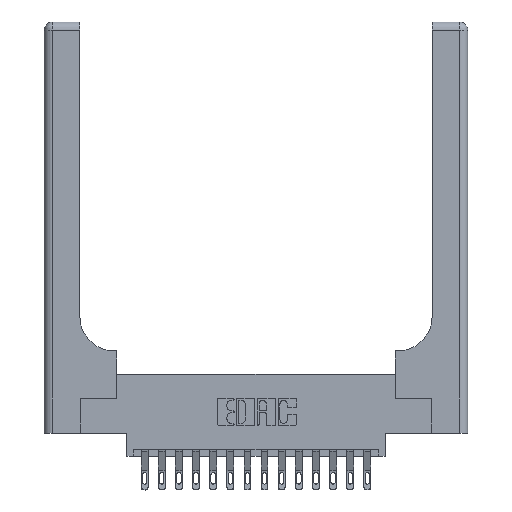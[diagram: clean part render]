
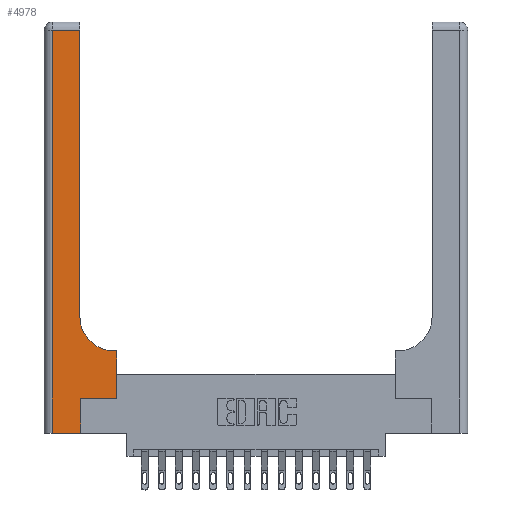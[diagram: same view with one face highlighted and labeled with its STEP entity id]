
A CAD part, top view. The second image highlights one B-rep face of the part: STEP entity #4978.
In plain terms, the highlighted planar face has unit normal (0, 0, 1).
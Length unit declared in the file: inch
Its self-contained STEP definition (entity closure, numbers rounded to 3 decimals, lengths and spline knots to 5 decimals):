
#12 = CARTESIAN_POINT ( 'NONE',  ( 0.26, 2.94, 0.37 ) ) ;
#31 = CARTESIAN_POINT ( 'NONE',  ( 0.26, 3., 0.37 ) ) ;
#469 = VERTEX_POINT ( 'NONE', #12 ) ;
#737 = ORIENTED_EDGE ( 'NONE', *, *, #15162, .T. ) ;
#1113 = VECTOR ( 'NONE', #2890, 39.37008 ) ;
#1508 = DIRECTION ( 'NONE',  ( 0., 1., 0. ) ) ;
#2030 = DIRECTION ( 'NONE',  ( -1., 0., 0. ) ) ;
#2580 = CARTESIAN_POINT ( 'NONE',  ( 0., 2.94, 0.37 ) ) ;
#2603 = VECTOR ( 'NONE', #15039, 39.37008 ) ;
#2890 = DIRECTION ( 'NONE',  ( 1., 0., 0. ) ) ;
#2992 = CARTESIAN_POINT ( 'NONE',  ( 0.528, 0.25, 0.37 ) ) ;
#3216 = VERTEX_POINT ( 'NONE', #11902 ) ;
#3473 = VERTEX_POINT ( 'NONE', #8165 ) ;
#3650 = EDGE_CURVE ( 'NONE', #15728, #469, #12330, .T. ) ;
#3864 = CARTESIAN_POINT ( 'NONE',  ( 0.26, 0.85, 0.37 ) ) ;
#4078 = VECTOR ( 'NONE', #12043, 39.37008 ) ;
#4079 = DIRECTION ( 'NONE',  ( -1., 0., 0. ) ) ;
#4214 = CARTESIAN_POINT ( 'NONE',  ( 0.528, 0.25, 0.37 ) ) ;
#4428 = VERTEX_POINT ( 'NONE', #9135 ) ;
#4525 = LINE ( 'NONE', #2580, #15442 ) ;
#4595 = AXIS2_PLACEMENT_3D ( 'NONE', #5331, #15278, #6759 ) ;
#4690 = PLANE ( 'NONE',  #7529 ) ;
#4805 = VECTOR ( 'NONE', #6976, 39.37008 ) ;
#4978 = ADVANCED_FACE ( 'NONE', ( #9402 ), #4690, .F. ) ;
#5121 = EDGE_CURVE ( 'NONE', #3216, #15539, #7165, .T. ) ;
#5331 = CARTESIAN_POINT ( 'NONE',  ( 0.51, 0.85, 0.37 ) ) ;
#5892 = EDGE_CURVE ( 'NONE', #11147, #3216, #17343, .T. ) ;
#5900 = ORIENTED_EDGE ( 'NONE', *, *, #14709, .T. ) ;
#6041 = VECTOR ( 'NONE', #11325, 39.37008 ) ;
#6281 = CARTESIAN_POINT ( 'NONE',  ( 0.51, 0.6, 0.37 ) ) ;
#6331 = CARTESIAN_POINT ( 'NONE',  ( 0.06, 3., 0.37 ) ) ;
#6537 = EDGE_CURVE ( 'NONE', #8228, #11248, #8812, .T. ) ;
#6759 = DIRECTION ( 'NONE',  ( 1., 0., 0. ) ) ;
#6817 = EDGE_CURVE ( 'NONE', #3473, #11147, #8582, .T. ) ;
#6976 = DIRECTION ( 'NONE',  ( 1., 0., 0. ) ) ;
#7165 = LINE ( 'NONE', #7799, #10519 ) ;
#7529 = AXIS2_PLACEMENT_3D ( 'NONE', #16071, #7547, #17464 ) ;
#7547 = DIRECTION ( 'NONE',  ( 0., 0., -1. ) ) ;
#7799 = CARTESIAN_POINT ( 'NONE',  ( 0.26, 0.6, 0.37 ) ) ;
#8065 = ORIENTED_EDGE ( 'NONE', *, *, #17404, .T. ) ;
#8165 = CARTESIAN_POINT ( 'NONE',  ( 0.265, 0.25, 0.37 ) ) ;
#8228 = VERTEX_POINT ( 'NONE', #14720 ) ;
#8582 = LINE ( 'NONE', #16906, #4805 ) ;
#8812 = LINE ( 'NONE', #15780, #1113 ) ;
#9135 = CARTESIAN_POINT ( 'NONE',  ( 0.06, 2.94, 0.37 ) ) ;
#9336 = CIRCLE ( 'NONE', #4595, 0.25 ) ;
#9402 = FACE_OUTER_BOUND ( 'NONE', #16044, .T. ) ;
#10519 = VECTOR ( 'NONE', #2030, 39.37008 ) ;
#11147 = VERTEX_POINT ( 'NONE', #2992 ) ;
#11229 = ORIENTED_EDGE ( 'NONE', *, *, #5892, .T. ) ;
#11248 = VERTEX_POINT ( 'NONE', #11810 ) ;
#11325 = DIRECTION ( 'NONE',  ( 0., 1., 0. ) ) ;
#11666 = LINE ( 'NONE', #6331, #4078 ) ;
#11810 = CARTESIAN_POINT ( 'NONE',  ( 0.265, 0., 0.37 ) ) ;
#11887 = VECTOR ( 'NONE', #1508, 39.37008 ) ;
#11902 = CARTESIAN_POINT ( 'NONE',  ( 0.528, 0.6, 0.37 ) ) ;
#11936 = EDGE_CURVE ( 'NONE', #15539, #15728, #9336, .T. ) ;
#12043 = DIRECTION ( 'NONE',  ( 0., -1., 0. ) ) ;
#12330 = LINE ( 'NONE', #31, #11887 ) ;
#13354 = ORIENTED_EDGE ( 'NONE', *, *, #11936, .T. ) ;
#13467 = ORIENTED_EDGE ( 'NONE', *, *, #5121, .T. ) ;
#14709 = EDGE_CURVE ( 'NONE', #4428, #8228, #11666, .T. ) ;
#14720 = CARTESIAN_POINT ( 'NONE',  ( 0.06, 0., 0.37 ) ) ;
#15039 = DIRECTION ( 'NONE',  ( 0., 1., 0. ) ) ;
#15162 = EDGE_CURVE ( 'NONE', #469, #4428, #4525, .T. ) ;
#15278 = DIRECTION ( 'NONE',  ( 0., 0., -1. ) ) ;
#15442 = VECTOR ( 'NONE', #4079, 39.37008 ) ;
#15539 = VERTEX_POINT ( 'NONE', #6281 ) ;
#15728 = VERTEX_POINT ( 'NONE', #3864 ) ;
#15780 = CARTESIAN_POINT ( 'NONE',  ( 0., 0., 0.37 ) ) ;
#16044 = EDGE_LOOP ( 'NONE', ( #17726, #737, #5900, #16501, #8065, #17897, #11229, #13467, #13354 ) ) ;
#16071 = CARTESIAN_POINT ( 'NONE',  ( 0., 3., 0.37 ) ) ;
#16501 = ORIENTED_EDGE ( 'NONE', *, *, #6537, .T. ) ;
#16906 = CARTESIAN_POINT ( 'NONE',  ( 0.265, 0.25, 0.37 ) ) ;
#17343 = LINE ( 'NONE', #4214, #6041 ) ;
#17354 = LINE ( 'NONE', #17852, #2603 ) ;
#17404 = EDGE_CURVE ( 'NONE', #11248, #3473, #17354, .T. ) ;
#17464 = DIRECTION ( 'NONE',  ( -1., 0., 0. ) ) ;
#17726 = ORIENTED_EDGE ( 'NONE', *, *, #3650, .T. ) ;
#17852 = CARTESIAN_POINT ( 'NONE',  ( 0.265, 0., 0.37 ) ) ;
#17897 = ORIENTED_EDGE ( 'NONE', *, *, #6817, .T. ) ;
